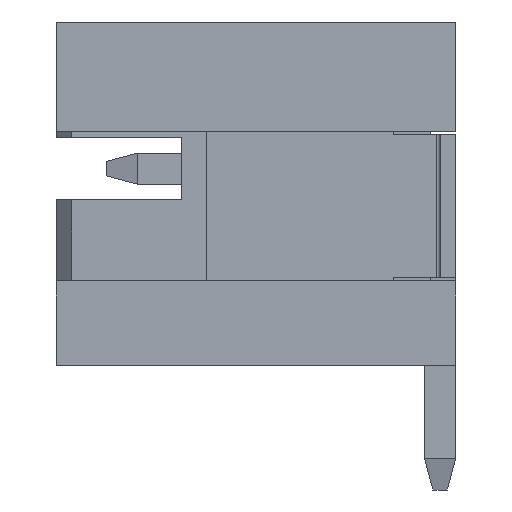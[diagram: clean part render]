
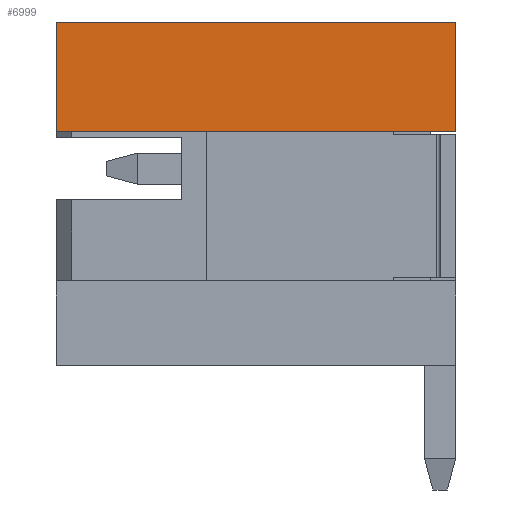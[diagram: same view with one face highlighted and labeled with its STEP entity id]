
A CAD part, left-side view. The second image highlights one B-rep face of the part: STEP entity #6999.
In plain terms, the highlighted planar face has unit normal (-1, 0, 0).
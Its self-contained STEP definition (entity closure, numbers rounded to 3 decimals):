
#415 = EDGE_CURVE ( 'NONE', #7251, #597, #2877, .T. ) ;
#597 = VERTEX_POINT ( 'NONE', #2043 ) ;
#737 = ORIENTED_EDGE ( 'NONE', *, *, #415, .F. ) ;
#920 = LINE ( 'NONE', #6733, #3442 ) ;
#1394 = ORIENTED_EDGE ( 'NONE', *, *, #5528, .F. ) ;
#1512 = EDGE_CURVE ( 'NONE', #7593, #7251, #4829, .T. ) ;
#1744 = CARTESIAN_POINT ( 'NONE',  ( -3., 0., 0.6 ) ) ;
#1963 = FACE_OUTER_BOUND ( 'NONE', #2181, .T. ) ;
#2043 = CARTESIAN_POINT ( 'NONE',  ( -3., 0., 2.35 ) ) ;
#2181 = EDGE_LOOP ( 'NONE', ( #5889, #1394, #6387, #737 ) ) ;
#2877 = LINE ( 'NONE', #5619, #4556 ) ;
#2886 = PLANE ( 'NONE',  #6617 ) ;
#2941 = CARTESIAN_POINT ( 'NONE',  ( -3., 0., 0.6 ) ) ;
#3316 = LINE ( 'NONE', #2941, #8248 ) ;
#3442 = VECTOR ( 'NONE', #9041, 1000. ) ;
#3519 = CARTESIAN_POINT ( 'NONE',  ( -3., 6.4, 0.6 ) ) ;
#4372 = CARTESIAN_POINT ( 'NONE',  ( -3., 0., 0. ) ) ;
#4556 = VECTOR ( 'NONE', #6521, 1000. ) ;
#4589 = CARTESIAN_POINT ( 'NONE',  ( -3., 6.4, 2.35 ) ) ;
#4829 = LINE ( 'NONE', #4589, #6627 ) ;
#5415 = CARTESIAN_POINT ( 'NONE',  ( -3., 6.4, 2.35 ) ) ;
#5528 = EDGE_CURVE ( 'NONE', #7763, #7593, #3316, .T. ) ;
#5619 = CARTESIAN_POINT ( 'NONE',  ( -3., 6.4, 2.35 ) ) ;
#5889 = ORIENTED_EDGE ( 'NONE', *, *, #1512, .F. ) ;
#6033 = DIRECTION ( 'NONE',  ( 0., 0., 1. ) ) ;
#6387 = ORIENTED_EDGE ( 'NONE', *, *, #9509, .F. ) ;
#6521 = DIRECTION ( 'NONE',  ( 0., -1., 0. ) ) ;
#6617 = AXIS2_PLACEMENT_3D ( 'NONE', #4372, #9757, #9081 ) ;
#6627 = VECTOR ( 'NONE', #6033, 1000. ) ;
#6733 = CARTESIAN_POINT ( 'NONE',  ( -3., 0., 2.35 ) ) ;
#6999 = ADVANCED_FACE ( 'NONE', ( #1963 ), #2886, .F. ) ;
#7251 = VERTEX_POINT ( 'NONE', #5415 ) ;
#7593 = VERTEX_POINT ( 'NONE', #3519 ) ;
#7763 = VERTEX_POINT ( 'NONE', #1744 ) ;
#8248 = VECTOR ( 'NONE', #8294, 1000. ) ;
#8294 = DIRECTION ( 'NONE',  ( 0., 1., 0. ) ) ;
#9041 = DIRECTION ( 'NONE',  ( 0., 0., -1. ) ) ;
#9081 = DIRECTION ( 'NONE',  ( 0., 0., -1. ) ) ;
#9509 = EDGE_CURVE ( 'NONE', #597, #7763, #920, .T. ) ;
#9757 = DIRECTION ( 'NONE',  ( 1., 0., 0. ) ) ;
